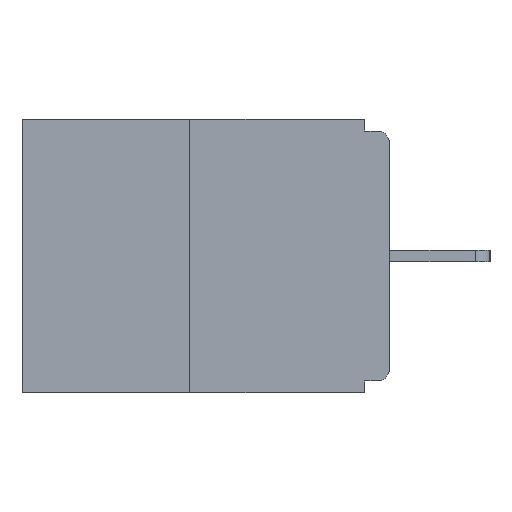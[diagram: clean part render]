
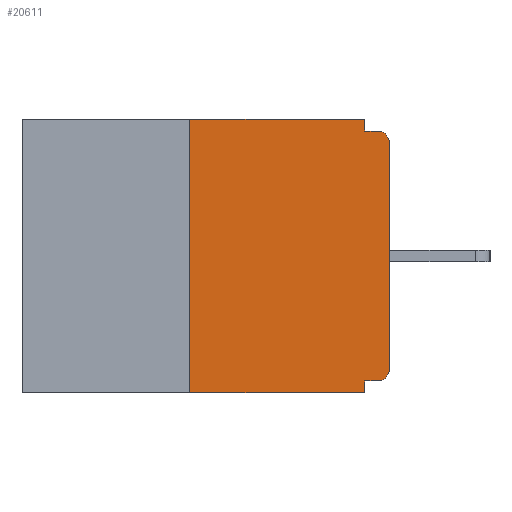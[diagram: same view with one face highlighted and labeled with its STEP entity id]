
A CAD part, left-side view. The second image highlights one B-rep face of the part: STEP entity #20611.
In plain terms, the highlighted planar face has unit normal (-1, 0, 0).
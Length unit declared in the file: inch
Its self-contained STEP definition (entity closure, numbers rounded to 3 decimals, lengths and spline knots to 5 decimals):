
#77 = ORIENTED_EDGE ( 'NONE', *, *, #7377, .T. ) ;
#829 = AXIS2_PLACEMENT_3D ( 'NONE', #20761, #10033, #22554 ) ;
#1286 = ORIENTED_EDGE ( 'NONE', *, *, #1764, .T. ) ;
#1596 = CARTESIAN_POINT ( 'NONE',  ( 0., 0.25, -0.343 ) ) ;
#1738 = VERTEX_POINT ( 'NONE', #1596 ) ;
#1764 = EDGE_CURVE ( 'NONE', #4385, #8542, #17077, .T. ) ;
#1936 = DIRECTION ( 'NONE',  ( 0., 0., 1. ) ) ;
#2608 = FACE_OUTER_BOUND ( 'NONE', #12891, .T. ) ;
#2739 = LINE ( 'NONE', #5513, #11853 ) ;
#3049 = LINE ( 'NONE', #8733, #12172 ) ;
#4180 = CARTESIAN_POINT ( 'NONE',  ( 0., 0.031, -0.343 ) ) ;
#4385 = VERTEX_POINT ( 'NONE', #9911 ) ;
#4533 = CARTESIAN_POINT ( 'NONE',  ( 0., 0.015, -0.328 ) ) ;
#4552 = CARTESIAN_POINT ( 'NONE',  ( 0., 0.015, -0.015 ) ) ;
#4893 = LINE ( 'NONE', #8549, #9723 ) ;
#5312 = AXIS2_PLACEMENT_3D ( 'NONE', #5333, #5501, #5408 ) ;
#5333 = CARTESIAN_POINT ( 'NONE',  ( 0., 0.015, -0.03 ) ) ;
#5408 = DIRECTION ( 'NONE',  ( 0., 0., -1. ) ) ;
#5501 = DIRECTION ( 'NONE',  ( -1., 0., 0. ) ) ;
#5513 = CARTESIAN_POINT ( 'NONE',  ( 0., 0., 0. ) ) ;
#5539 = DIRECTION ( 'NONE',  ( 0., -1., 0. ) ) ;
#5955 = EDGE_CURVE ( 'NONE', #19437, #8542, #3049, .T. ) ;
#6255 = VERTEX_POINT ( 'NONE', #21311 ) ;
#6443 = EDGE_CURVE ( 'NONE', #1738, #6255, #6709, .T. ) ;
#6514 = CARTESIAN_POINT ( 'NONE',  ( 0., 0.031, -0.015 ) ) ;
#6709 = LINE ( 'NONE', #7818, #10991 ) ;
#6727 = VECTOR ( 'NONE', #5539, 39.37008 ) ;
#6739 = DIRECTION ( 'NONE',  ( 0., -1., 0. ) ) ;
#6799 = VERTEX_POINT ( 'NONE', #13849 ) ;
#6996 = CARTESIAN_POINT ( 'NONE',  ( 0., 0., -0.313 ) ) ;
#7016 = ORIENTED_EDGE ( 'NONE', *, *, #16705, .F. ) ;
#7250 = EDGE_CURVE ( 'NONE', #13120, #23123, #21576, .T. ) ;
#7288 = VERTEX_POINT ( 'NONE', #4533 ) ;
#7377 = EDGE_CURVE ( 'NONE', #7288, #22259, #18762, .T. ) ;
#7590 = ORIENTED_EDGE ( 'NONE', *, *, #6443, .F. ) ;
#7757 = DIRECTION ( 'NONE',  ( 0., 0., 1. ) ) ;
#7818 = CARTESIAN_POINT ( 'NONE',  ( 0., 0.25, 0. ) ) ;
#8006 = VECTOR ( 'NONE', #22488, 39.37008 ) ;
#8144 = PLANE ( 'NONE',  #829 ) ;
#8389 = VECTOR ( 'NONE', #22390, 39.37008 ) ;
#8434 = DIRECTION ( 'NONE',  ( -1., 0., 0. ) ) ;
#8450 = LINE ( 'NONE', #21585, #22744 ) ;
#8542 = VERTEX_POINT ( 'NONE', #4552 ) ;
#8549 = CARTESIAN_POINT ( 'NONE',  ( 0., 0., -0.328 ) ) ;
#8729 = ORIENTED_EDGE ( 'NONE', *, *, #20145, .F. ) ;
#8733 = CARTESIAN_POINT ( 'NONE',  ( 0., 0., -0.015 ) ) ;
#9723 = VECTOR ( 'NONE', #10369, 39.37008 ) ;
#9911 = CARTESIAN_POINT ( 'NONE',  ( 0., 0., -0.03 ) ) ;
#10033 = DIRECTION ( 'NONE',  ( 1., 0., 0. ) ) ;
#10134 = CARTESIAN_POINT ( 'NONE',  ( 0., 0.031, -0.328 ) ) ;
#10369 = DIRECTION ( 'NONE',  ( 0., 1., 0. ) ) ;
#10991 = VECTOR ( 'NONE', #7757, 39.37008 ) ;
#11562 = EDGE_CURVE ( 'NONE', #6799, #19437, #17550, .T. ) ;
#11727 = CARTESIAN_POINT ( 'NONE',  ( 0., 0.031, -0.343 ) ) ;
#11853 = VECTOR ( 'NONE', #1936, 39.37008 ) ;
#12172 = VECTOR ( 'NONE', #6739, 39.37008 ) ;
#12431 = ORIENTED_EDGE ( 'NONE', *, *, #16741, .T. ) ;
#12725 = LINE ( 'NONE', #16372, #6727 ) ;
#12891 = EDGE_LOOP ( 'NONE', ( #7016, #7590, #12431, #21921, #8729, #77, #14701, #1286, #16348, #21941 ) ) ;
#13120 = VERTEX_POINT ( 'NONE', #10134 ) ;
#13849 = CARTESIAN_POINT ( 'NONE',  ( 0., 0.031, 0. ) ) ;
#14701 = ORIENTED_EDGE ( 'NONE', *, *, #17365, .T. ) ;
#16348 = ORIENTED_EDGE ( 'NONE', *, *, #5955, .F. ) ;
#16372 = CARTESIAN_POINT ( 'NONE',  ( 0., 0.46, -0.343 ) ) ;
#16705 = EDGE_CURVE ( 'NONE', #6255, #6799, #8450, .T. ) ;
#16741 = EDGE_CURVE ( 'NONE', #1738, #23123, #12725, .T. ) ;
#17077 = CIRCLE ( 'NONE', #5312, 0.015 ) ;
#17365 = EDGE_CURVE ( 'NONE', #22259, #4385, #2739, .T. ) ;
#17550 = LINE ( 'NONE', #20684, #8006 ) ;
#18762 = CIRCLE ( 'NONE', #22113, 0.015 ) ;
#19163 = CARTESIAN_POINT ( 'NONE',  ( 0., 0.015, -0.313 ) ) ;
#19437 = VERTEX_POINT ( 'NONE', #6514 ) ;
#20145 = EDGE_CURVE ( 'NONE', #7288, #13120, #4893, .T. ) ;
#20611 = ADVANCED_FACE ( 'NONE', ( #2608 ), #8144, .F. ) ;
#20684 = CARTESIAN_POINT ( 'NONE',  ( 0., 0.031, 0. ) ) ;
#20761 = CARTESIAN_POINT ( 'NONE',  ( 0., 0.46, 0. ) ) ;
#20960 = DIRECTION ( 'NONE',  ( 0., 0., -1. ) ) ;
#21311 = CARTESIAN_POINT ( 'NONE',  ( 0., 0.25, 0. ) ) ;
#21503 = DIRECTION ( 'NONE',  ( 0., -1., 0. ) ) ;
#21576 = LINE ( 'NONE', #11727, #8389 ) ;
#21585 = CARTESIAN_POINT ( 'NONE',  ( 0., 0.46, 0. ) ) ;
#21921 = ORIENTED_EDGE ( 'NONE', *, *, #7250, .F. ) ;
#21941 = ORIENTED_EDGE ( 'NONE', *, *, #11562, .F. ) ;
#22113 = AXIS2_PLACEMENT_3D ( 'NONE', #19163, #8434, #20960 ) ;
#22259 = VERTEX_POINT ( 'NONE', #6996 ) ;
#22390 = DIRECTION ( 'NONE',  ( 0., 0., -1. ) ) ;
#22488 = DIRECTION ( 'NONE',  ( 0., 0., -1. ) ) ;
#22554 = DIRECTION ( 'NONE',  ( 0., 0., -1. ) ) ;
#22744 = VECTOR ( 'NONE', #21503, 39.37008 ) ;
#23123 = VERTEX_POINT ( 'NONE', #4180 ) ;
